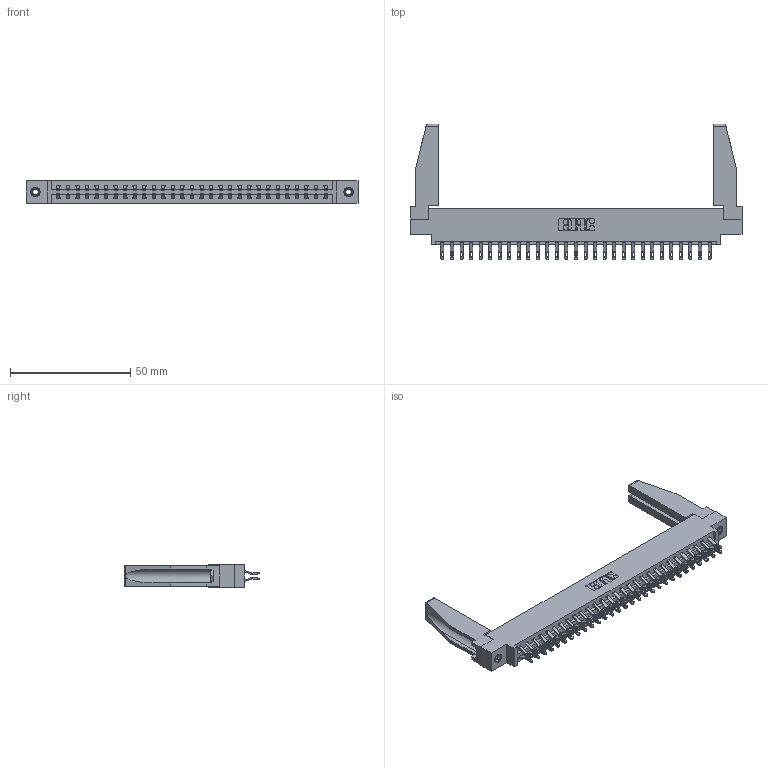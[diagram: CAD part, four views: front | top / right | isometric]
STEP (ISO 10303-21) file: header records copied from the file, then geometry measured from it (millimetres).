
FILE_DESCRIPTION (( 'STEP AP203' ), '1' );
FILE_NAME ('337-058-555-878.STEP', '2019-10-11T20:59:25', ( '' ), ( '' ), 'SwSTEP 2.0', 'SolidWorks 2016', '' );
FILE_SCHEMA (( 'CONFIG_CONTROL_DESIGN' ));
Length unit declared in the file: inch
Products named in the file (5): 337 Part_0.170 Offset - 0.156 Dia-TI; 337-058-555-878; 345-292-001_555 Tail; 307-220-078; 345-250-001_345-250-001-102
Assembly tree (63 placements, depth 2):
  337-058-555-878
    337 Part_0.170 Offset - 0.156 Dia-TI
    345-292-001_555 Tail  x58
    345-250-001_345-250-001-102  x2
    307-220-078  x2
Bounding box: 137.92 x 56.27 x 9.4 mm (x, y, z)
Volume: 18406.3 mm3; surface area: 20739.9 mm2
Topology: 63 solids, 63 shells, 3728 faces, 11615 edges, 7734 vertices
Faces by surface type: plane 2246, cylinder 1466, cone 12, torus 4
Entity records: 27064 total; most frequent: CARTESIAN_POINT 4606, ORIENTED_EDGE 4468, DIRECTION 3918, EDGE_CURVE 2234, LINE 2048, VECTOR 2048, VERTEX_POINT 1484, AXIS2_PLACEMENT_3D 935
